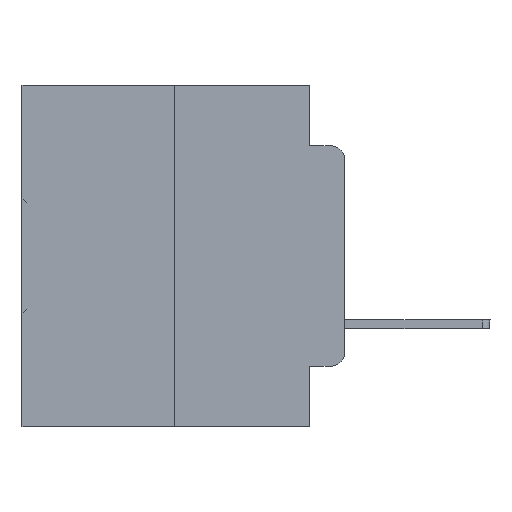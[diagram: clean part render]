
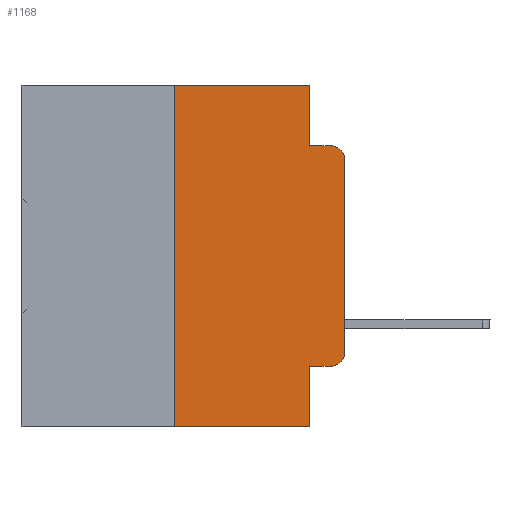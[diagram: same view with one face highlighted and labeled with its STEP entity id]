
A CAD part, left-side view. The second image highlights one B-rep face of the part: STEP entity #1168.
In plain terms, the highlighted planar face has unit normal (-1, 0, 0).
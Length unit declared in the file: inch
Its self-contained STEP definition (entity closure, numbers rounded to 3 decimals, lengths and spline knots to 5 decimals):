
#135 = ORIENTED_EDGE ( 'NONE', *, *, #5892, .T. ) ;
#212 = CARTESIAN_POINT ( 'NONE',  ( 0., 0.25, -0.5 ) ) ;
#1168 = ADVANCED_FACE ( 'NONE', ( #34053 ), #16056, .F. ) ;
#1277 = EDGE_CURVE ( 'NONE', #12384, #22960, #16388, .T. ) ;
#1614 = VERTEX_POINT ( 'NONE', #3509 ) ;
#1615 = VERTEX_POINT ( 'NONE', #27407 ) ;
#1708 = VECTOR ( 'NONE', #6648, 39.37008 ) ;
#2209 = AXIS2_PLACEMENT_3D ( 'NONE', #26618, #29027, #2896 ) ;
#2388 = DIRECTION ( 'NONE',  ( 0., -1., 0. ) ) ;
#2896 = DIRECTION ( 'NONE',  ( 0., 0., -1. ) ) ;
#3509 = CARTESIAN_POINT ( 'NONE',  ( 0., 0.02, -0.0885 ) ) ;
#3676 = DIRECTION ( 'NONE',  ( 0., 0., -1. ) ) ;
#3684 = VECTOR ( 'NONE', #25739, 39.37008 ) ;
#4583 = CARTESIAN_POINT ( 'NONE',  ( 0., 0.473, -0.5 ) ) ;
#5892 = EDGE_CURVE ( 'NONE', #1615, #1614, #10392, .T. ) ;
#6648 = DIRECTION ( 'NONE',  ( 0., -1., 0. ) ) ;
#7002 = DIRECTION ( 'NONE',  ( 0., 0., 1. ) ) ;
#7777 = EDGE_LOOP ( 'NONE', ( #20125, #135, #15247, #25224, #30970, #32347, #30473, #28329, #13116, #13448 ) ) ;
#8660 = LINE ( 'NONE', #11441, #30652 ) ;
#9767 = LINE ( 'NONE', #30702, #28483 ) ;
#10086 = EDGE_CURVE ( 'NONE', #22960, #30241, #15218, .T. ) ;
#10392 = CIRCLE ( 'NONE', #22542, 0.02 ) ;
#11441 = CARTESIAN_POINT ( 'NONE',  ( 0., 0.051, 0. ) ) ;
#11766 = EDGE_CURVE ( 'NONE', #31864, #21991, #13102, .T. ) ;
#12007 = CARTESIAN_POINT ( 'NONE',  ( 0., 0.051, -0.0885 ) ) ;
#12384 = VERTEX_POINT ( 'NONE', #212 ) ;
#12437 = VERTEX_POINT ( 'NONE', #20114 ) ;
#12791 = AXIS2_PLACEMENT_3D ( 'NONE', #24630, #21691, #16511 ) ;
#13102 = LINE ( 'NONE', #31441, #3684 ) ;
#13116 = ORIENTED_EDGE ( 'NONE', *, *, #11766, .T. ) ;
#13448 = ORIENTED_EDGE ( 'NONE', *, *, #17880, .T. ) ;
#13451 = DIRECTION ( 'NONE',  ( 0., 0., -1. ) ) ;
#15126 = EDGE_CURVE ( 'NONE', #12384, #12437, #22912, .T. ) ;
#15218 = LINE ( 'NONE', #31635, #19703 ) ;
#15247 = ORIENTED_EDGE ( 'NONE', *, *, #17961, .F. ) ;
#15282 = LINE ( 'NONE', #12007, #1708 ) ;
#15380 = CARTESIAN_POINT ( 'NONE',  ( 0., 0.02, -0.4115 ) ) ;
#16056 = PLANE ( 'NONE',  #2209 ) ;
#16388 = LINE ( 'NONE', #32818, #29414 ) ;
#16511 = DIRECTION ( 'NONE',  ( 0., 0., -1. ) ) ;
#17880 = EDGE_CURVE ( 'NONE', #21991, #34157, #27709, .T. ) ;
#17961 = EDGE_CURVE ( 'NONE', #25195, #1614, #15282, .T. ) ;
#18018 = VECTOR ( 'NONE', #13451, 39.37008 ) ;
#18895 = DIRECTION ( 'NONE',  ( -1., 0., 0. ) ) ;
#19200 = CARTESIAN_POINT ( 'NONE',  ( 0., 0.25, 0. ) ) ;
#19300 = CARTESIAN_POINT ( 'NONE',  ( 0., 0.051, -0.0885 ) ) ;
#19703 = VECTOR ( 'NONE', #2388, 39.37008 ) ;
#20114 = CARTESIAN_POINT ( 'NONE',  ( 0., 0.051, -0.5 ) ) ;
#20125 = ORIENTED_EDGE ( 'NONE', *, *, #24050, .T. ) ;
#20662 = DIRECTION ( 'NONE',  ( 0., -1., 0. ) ) ;
#20898 = CARTESIAN_POINT ( 'NONE',  ( 0., 0.051, 0. ) ) ;
#21691 = DIRECTION ( 'NONE',  ( -1., 0., 0. ) ) ;
#21991 = VERTEX_POINT ( 'NONE', #15380 ) ;
#22466 = CARTESIAN_POINT ( 'NONE',  ( 0., 0., -0.3915 ) ) ;
#22542 = AXIS2_PLACEMENT_3D ( 'NONE', #27564, #18895, #3676 ) ;
#22912 = LINE ( 'NONE', #4583, #33637 ) ;
#22960 = VERTEX_POINT ( 'NONE', #19200 ) ;
#24050 = EDGE_CURVE ( 'NONE', #34157, #1615, #9767, .T. ) ;
#24630 = CARTESIAN_POINT ( 'NONE',  ( 0., 0.02, -0.3915 ) ) ;
#25195 = VERTEX_POINT ( 'NONE', #19300 ) ;
#25224 = ORIENTED_EDGE ( 'NONE', *, *, #29772, .F. ) ;
#25739 = DIRECTION ( 'NONE',  ( 0., -1., 0. ) ) ;
#26286 = CARTESIAN_POINT ( 'NONE',  ( 0., 0.051, 0. ) ) ;
#26442 = LINE ( 'NONE', #20898, #18018 ) ;
#26527 = EDGE_CURVE ( 'NONE', #31864, #12437, #8660, .T. ) ;
#26618 = CARTESIAN_POINT ( 'NONE',  ( 0., 0.473, 0. ) ) ;
#27129 = DIRECTION ( 'NONE',  ( 0., 0., 1. ) ) ;
#27353 = DIRECTION ( 'NONE',  ( 0., 0., -1. ) ) ;
#27407 = CARTESIAN_POINT ( 'NONE',  ( 0., 0., -0.1085 ) ) ;
#27564 = CARTESIAN_POINT ( 'NONE',  ( 0., 0.02, -0.1085 ) ) ;
#27709 = CIRCLE ( 'NONE', #12791, 0.02 ) ;
#28329 = ORIENTED_EDGE ( 'NONE', *, *, #26527, .F. ) ;
#28483 = VECTOR ( 'NONE', #7002, 39.37008 ) ;
#29027 = DIRECTION ( 'NONE',  ( 1., 0., 0. ) ) ;
#29414 = VECTOR ( 'NONE', #27129, 39.37008 ) ;
#29772 = EDGE_CURVE ( 'NONE', #30241, #25195, #26442, .T. ) ;
#30241 = VERTEX_POINT ( 'NONE', #26286 ) ;
#30473 = ORIENTED_EDGE ( 'NONE', *, *, #15126, .T. ) ;
#30652 = VECTOR ( 'NONE', #27353, 39.37008 ) ;
#30702 = CARTESIAN_POINT ( 'NONE',  ( 0., 0., 0. ) ) ;
#30970 = ORIENTED_EDGE ( 'NONE', *, *, #10086, .F. ) ;
#31281 = CARTESIAN_POINT ( 'NONE',  ( 0., 0.051, -0.4115 ) ) ;
#31441 = CARTESIAN_POINT ( 'NONE',  ( 0., 0.051, -0.4115 ) ) ;
#31635 = CARTESIAN_POINT ( 'NONE',  ( 0., 0.473, 0. ) ) ;
#31864 = VERTEX_POINT ( 'NONE', #31281 ) ;
#32347 = ORIENTED_EDGE ( 'NONE', *, *, #1277, .F. ) ;
#32818 = CARTESIAN_POINT ( 'NONE',  ( 0., 0.25, 0. ) ) ;
#33637 = VECTOR ( 'NONE', #20662, 39.37008 ) ;
#34053 = FACE_OUTER_BOUND ( 'NONE', #7777, .T. ) ;
#34157 = VERTEX_POINT ( 'NONE', #22466 ) ;
